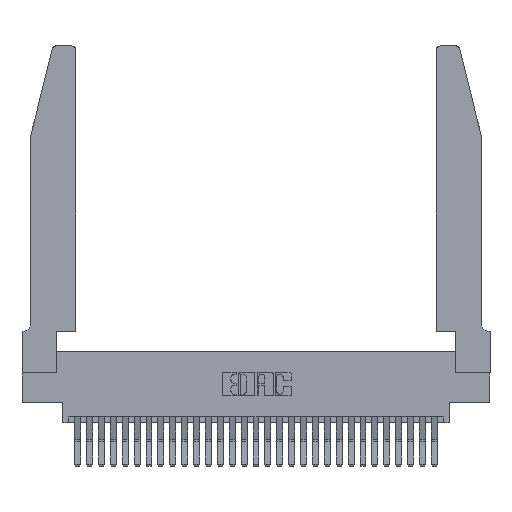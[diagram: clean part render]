
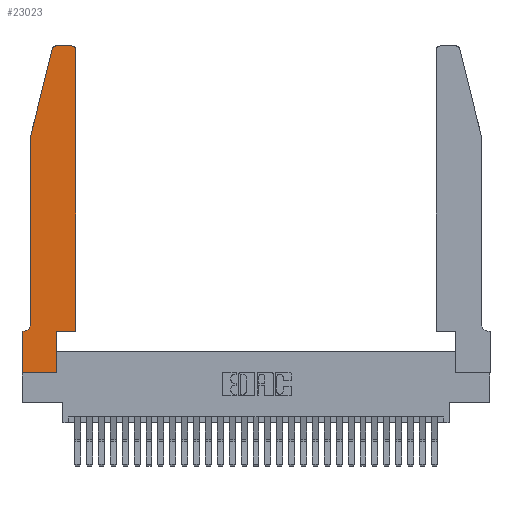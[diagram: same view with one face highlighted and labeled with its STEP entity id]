
A CAD part, top view. The second image highlights one B-rep face of the part: STEP entity #23023.
In plain terms, the highlighted planar face has unit normal (0, 0, 1).
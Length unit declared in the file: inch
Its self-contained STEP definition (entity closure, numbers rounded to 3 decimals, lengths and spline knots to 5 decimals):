
#112 = LINE ( 'NONE', #3008, #18468 ) ;
#128 = LINE ( 'NONE', #11513, #871 ) ;
#251 = ORIENTED_EDGE ( 'NONE', *, *, #4950, .T. ) ;
#709 = LINE ( 'NONE', #25374, #25341 ) ;
#871 = VECTOR ( 'NONE', #25679, 39.37008 ) ;
#1616 = DIRECTION ( 'NONE',  ( -0.239, -0.971, 0. ) ) ;
#2019 = VERTEX_POINT ( 'NONE', #7868 ) ;
#2255 = DIRECTION ( 'NONE',  ( 1., 0., 0. ) ) ;
#3008 = CARTESIAN_POINT ( 'NONE',  ( 0.4505, 0.35, 0.37 ) ) ;
#3136 = CARTESIAN_POINT ( 'NONE',  ( 0.4505, 0.35, 0.37 ) ) ;
#3240 = DIRECTION ( 'NONE',  ( 0., 0., -1. ) ) ;
#3317 = LINE ( 'NONE', #20194, #26391 ) ;
#3346 = AXIS2_PLACEMENT_3D ( 'NONE', #27074, #12931, #29434 ) ;
#4027 = VECTOR ( 'NONE', #9561, 39.37008 ) ;
#4055 = ORIENTED_EDGE ( 'NONE', *, *, #17725, .T. ) ;
#4537 = EDGE_CURVE ( 'NONE', #18453, #18737, #28559, .T. ) ;
#4950 = EDGE_CURVE ( 'NONE', #30657, #18453, #23072, .T. ) ;
#6301 = ORIENTED_EDGE ( 'NONE', *, *, #25288, .T. ) ;
#7137 = CARTESIAN_POINT ( 'NONE',  ( 0.0755, 2., 0.37 ) ) ;
#7184 = VERTEX_POINT ( 'NONE', #23322 ) ;
#7211 = VECTOR ( 'NONE', #11332, 39.37008 ) ;
#7553 = EDGE_CURVE ( 'NONE', #18737, #11879, #15768, .T. ) ;
#7566 = CARTESIAN_POINT ( 'NONE',  ( 0.4505, 2.72, 0.37 ) ) ;
#7868 = CARTESIAN_POINT ( 'NONE',  ( 0.2865, 0., 0.37 ) ) ;
#8676 = VECTOR ( 'NONE', #26967, 39.37008 ) ;
#8944 = ORIENTED_EDGE ( 'NONE', *, *, #7553, .T. ) ;
#9561 = DIRECTION ( 'NONE',  ( 0., -1., 0. ) ) ;
#9730 = DIRECTION ( 'NONE',  ( 0., 0., 1. ) ) ;
#10806 = EDGE_CURVE ( 'NONE', #11879, #14347, #14067, .T. ) ;
#10920 = FACE_OUTER_BOUND ( 'NONE', #30402, .T. ) ;
#11332 = DIRECTION ( 'NONE',  ( 0., 1., 0. ) ) ;
#11513 = CARTESIAN_POINT ( 'NONE',  ( 0.2605, 2.75, 0.37 ) ) ;
#11544 = EDGE_CURVE ( 'NONE', #27832, #22301, #112, .T. ) ;
#11879 = VERTEX_POINT ( 'NONE', #18474 ) ;
#11936 = ORIENTED_EDGE ( 'NONE', *, *, #10806, .T. ) ;
#11977 = CARTESIAN_POINT ( 'NONE',  ( 0.2865, 0.35, 0.37 ) ) ;
#12701 = DIRECTION ( 'NONE',  ( 0., 1., 0. ) ) ;
#12820 = CARTESIAN_POINT ( 'NONE',  ( 0.0755, 0.35, 0.37 ) ) ;
#12931 = DIRECTION ( 'NONE',  ( 0., 0., 1. ) ) ;
#13771 = CARTESIAN_POINT ( 'NONE',  ( 0., 0., 0.37 ) ) ;
#14056 = VERTEX_POINT ( 'NONE', #7566 ) ;
#14067 = LINE ( 'NONE', #13771, #20382 ) ;
#14135 = AXIS2_PLACEMENT_3D ( 'NONE', #17578, #3240, #19976 ) ;
#14347 = VERTEX_POINT ( 'NONE', #20676 ) ;
#14981 = DIRECTION ( 'NONE',  ( 1., 0., 0. ) ) ;
#15451 = LINE ( 'NONE', #3136, #27982 ) ;
#15571 = AXIS2_PLACEMENT_3D ( 'NONE', #28348, #16629, #2255 ) ;
#15768 = LINE ( 'NONE', #12820, #8676 ) ;
#16071 = AXIS2_PLACEMENT_3D ( 'NONE', #23945, #9730, #26283 ) ;
#16629 = DIRECTION ( 'NONE',  ( 0., 0., 1. ) ) ;
#17141 = ORIENTED_EDGE ( 'NONE', *, *, #18029, .T. ) ;
#17384 = VERTEX_POINT ( 'NONE', #17796 ) ;
#17578 = CARTESIAN_POINT ( 'NONE',  ( 0.0055, 0.42, 0.37 ) ) ;
#17725 = EDGE_CURVE ( 'NONE', #22301, #14056, #15451, .T. ) ;
#17796 = CARTESIAN_POINT ( 'NONE',  ( 0.284, 2.75, 0.37 ) ) ;
#18029 = EDGE_CURVE ( 'NONE', #2019, #27832, #19881, .T. ) ;
#18277 = ORIENTED_EDGE ( 'NONE', *, *, #28981, .T. ) ;
#18453 = VERTEX_POINT ( 'NONE', #26914 ) ;
#18468 = VECTOR ( 'NONE', #14981, 39.37008 ) ;
#18474 = CARTESIAN_POINT ( 'NONE',  ( 0., 0.35, 0.37 ) ) ;
#18632 = ORIENTED_EDGE ( 'NONE', *, *, #11544, .T. ) ;
#18737 = VERTEX_POINT ( 'NONE', #27021 ) ;
#18893 = PLANE ( 'NONE',  #15571 ) ;
#18941 = EDGE_CURVE ( 'NONE', #7184, #30657, #709, .T. ) ;
#18986 = DIRECTION ( 'NONE',  ( 1., 0., 0. ) ) ;
#19747 = ORIENTED_EDGE ( 'NONE', *, *, #26221, .T. ) ;
#19881 = LINE ( 'NONE', #20792, #7211 ) ;
#19976 = DIRECTION ( 'NONE',  ( -1., 0., 0. ) ) ;
#20109 = ORIENTED_EDGE ( 'NONE', *, *, #4537, .T. ) ;
#20110 = CIRCLE ( 'NONE', #3346, 0.03 ) ;
#20194 = CARTESIAN_POINT ( 'NONE',  ( 0., 0., 0.37 ) ) ;
#20382 = VECTOR ( 'NONE', #27904, 39.37008 ) ;
#20676 = CARTESIAN_POINT ( 'NONE',  ( 0., 0., 0.37 ) ) ;
#20792 = CARTESIAN_POINT ( 'NONE',  ( 0.2865, 0.35, 0.37 ) ) ;
#20881 = EDGE_CURVE ( 'NONE', #24878, #17384, #128, .T. ) ;
#21569 = ORIENTED_EDGE ( 'NONE', *, *, #20881, .T. ) ;
#22301 = VERTEX_POINT ( 'NONE', #23515 ) ;
#22309 = CARTESIAN_POINT ( 'NONE',  ( 0.0755, 2., 0.37 ) ) ;
#23023 = ADVANCED_FACE ( 'NONE', ( #10920 ), #18893, .T. ) ;
#23072 = LINE ( 'NONE', #7137, #4027 ) ;
#23322 = CARTESIAN_POINT ( 'NONE',  ( 0.25487, 2.72718, 0.37 ) ) ;
#23515 = CARTESIAN_POINT ( 'NONE',  ( 0.4505, 0.35, 0.37 ) ) ;
#23945 = CARTESIAN_POINT ( 'NONE',  ( 0.4205, 2.72, 0.37 ) ) ;
#24878 = VERTEX_POINT ( 'NONE', #27606 ) ;
#25288 = EDGE_CURVE ( 'NONE', #17384, #7184, #20110, .T. ) ;
#25341 = VECTOR ( 'NONE', #1616, 39.37008 ) ;
#25374 = CARTESIAN_POINT ( 'NONE',  ( 0.0755, 2., 0.37 ) ) ;
#25679 = DIRECTION ( 'NONE',  ( -1., 0., 0. ) ) ;
#25970 = ORIENTED_EDGE ( 'NONE', *, *, #18941, .T. ) ;
#26221 = EDGE_CURVE ( 'NONE', #14347, #2019, #3317, .T. ) ;
#26283 = DIRECTION ( 'NONE',  ( 1., 0., 0. ) ) ;
#26391 = VECTOR ( 'NONE', #18986, 39.37008 ) ;
#26914 = CARTESIAN_POINT ( 'NONE',  ( 0.0755, 0.42, 0.37 ) ) ;
#26967 = DIRECTION ( 'NONE',  ( -1., 0., 0. ) ) ;
#27021 = CARTESIAN_POINT ( 'NONE',  ( 0.0055, 0.35, 0.37 ) ) ;
#27074 = CARTESIAN_POINT ( 'NONE',  ( 0.284, 2.72, 0.37 ) ) ;
#27606 = CARTESIAN_POINT ( 'NONE',  ( 0.4205, 2.75, 0.37 ) ) ;
#27832 = VERTEX_POINT ( 'NONE', #11977 ) ;
#27904 = DIRECTION ( 'NONE',  ( 0., -1., 0. ) ) ;
#27982 = VECTOR ( 'NONE', #12701, 39.37008 ) ;
#28348 = CARTESIAN_POINT ( 'NONE',  ( 0., 0.35, 0.37 ) ) ;
#28559 = CIRCLE ( 'NONE', #14135, 0.07 ) ;
#28821 = CIRCLE ( 'NONE', #16071, 0.03 ) ;
#28981 = EDGE_CURVE ( 'NONE', #14056, #24878, #28821, .T. ) ;
#29434 = DIRECTION ( 'NONE',  ( 1., 0., 0. ) ) ;
#30402 = EDGE_LOOP ( 'NONE', ( #21569, #6301, #25970, #251, #20109, #8944, #11936, #19747, #17141, #18632, #4055, #18277 ) ) ;
#30657 = VERTEX_POINT ( 'NONE', #22309 ) ;
